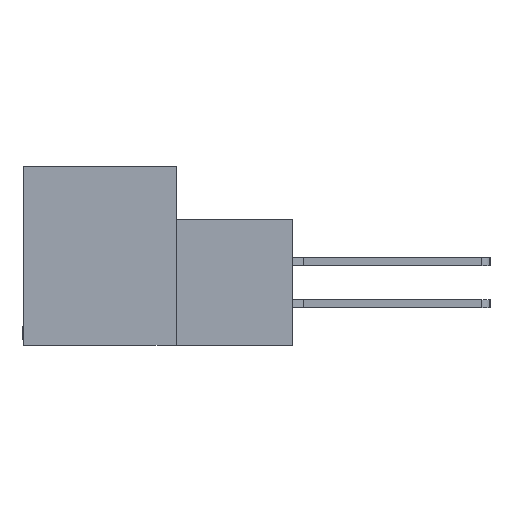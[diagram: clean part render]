
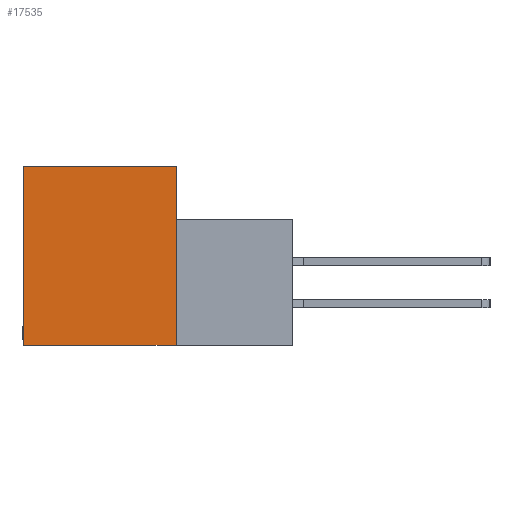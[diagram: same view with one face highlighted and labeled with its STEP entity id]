
A CAD part, left-side view. The second image highlights one B-rep face of the part: STEP entity #17535.
In plain terms, the highlighted planar face has unit normal (-1, 0, 0).
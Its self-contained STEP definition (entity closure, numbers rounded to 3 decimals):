
#2132 = CARTESIAN_POINT ( 'NONE',  ( 0., 0., 0. ) ) ;
#2180 = PLANE ( 'NONE',  #15298 ) ;
#3027 = LINE ( 'NONE', #12948, #30072 ) ;
#5950 = DIRECTION ( 'NONE',  ( 0., 0., 1. ) ) ;
#6859 = VECTOR ( 'NONE', #5950, 1000. ) ;
#7996 = ORIENTED_EDGE ( 'NONE', *, *, #42077, .F. ) ;
#8144 = EDGE_CURVE ( 'NONE', #14468, #37823, #18293, .T. ) ;
#9958 = CARTESIAN_POINT ( 'NONE',  ( 0., 11.506, -13.487 ) ) ;
#11693 = VECTOR ( 'NONE', #31197, 1000. ) ;
#12948 = CARTESIAN_POINT ( 'NONE',  ( 0., 11.506, 0. ) ) ;
#14468 = VERTEX_POINT ( 'NONE', #19724 ) ;
#15298 = AXIS2_PLACEMENT_3D ( 'NONE', #30407, #16075, #26586 ) ;
#16075 = DIRECTION ( 'NONE',  ( 1., 0., 0. ) ) ;
#16412 = CARTESIAN_POINT ( 'NONE',  ( 0., 11.506, 0. ) ) ;
#17535 = ADVANCED_FACE ( 'NONE', ( #27694 ), #2180, .F. ) ;
#18293 = LINE ( 'NONE', #23966, #11693 ) ;
#19724 = CARTESIAN_POINT ( 'NONE',  ( 0., 0., -13.487 ) ) ;
#22830 = CARTESIAN_POINT ( 'NONE',  ( 0., 0., 0. ) ) ;
#22903 = EDGE_CURVE ( 'NONE', #41998, #14468, #41013, .T. ) ;
#23903 = DIRECTION ( 'NONE',  ( 0., -1., 0. ) ) ;
#23966 = CARTESIAN_POINT ( 'NONE',  ( 0., -8.814, -13.487 ) ) ;
#26054 = DIRECTION ( 'NONE',  ( 0., 0., -1. ) ) ;
#26586 = DIRECTION ( 'NONE',  ( 0., 0., -1. ) ) ;
#27694 = FACE_OUTER_BOUND ( 'NONE', #45168, .T. ) ;
#30072 = VECTOR ( 'NONE', #23903, 1000. ) ;
#30407 = CARTESIAN_POINT ( 'NONE',  ( 0., 0., 0. ) ) ;
#31197 = DIRECTION ( 'NONE',  ( 0., 1., 0. ) ) ;
#31198 = EDGE_CURVE ( 'NONE', #37823, #35945, #32779, .T. ) ;
#31534 = ORIENTED_EDGE ( 'NONE', *, *, #8144, .F. ) ;
#32779 = LINE ( 'NONE', #44518, #6859 ) ;
#35945 = VERTEX_POINT ( 'NONE', #16412 ) ;
#37823 = VERTEX_POINT ( 'NONE', #9958 ) ;
#39423 = ORIENTED_EDGE ( 'NONE', *, *, #31198, .F. ) ;
#39714 = ORIENTED_EDGE ( 'NONE', *, *, #22903, .F. ) ;
#41013 = LINE ( 'NONE', #22830, #43237 ) ;
#41998 = VERTEX_POINT ( 'NONE', #2132 ) ;
#42077 = EDGE_CURVE ( 'NONE', #35945, #41998, #3027, .T. ) ;
#43237 = VECTOR ( 'NONE', #26054, 1000. ) ;
#44518 = CARTESIAN_POINT ( 'NONE',  ( 0., 11.506, -13.487 ) ) ;
#45168 = EDGE_LOOP ( 'NONE', ( #31534, #39714, #7996, #39423 ) ) ;
